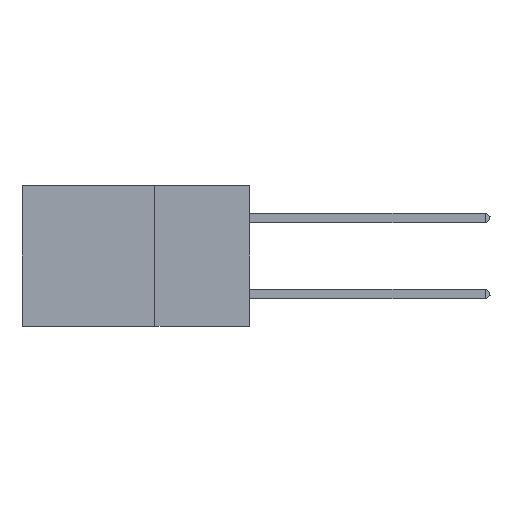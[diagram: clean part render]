
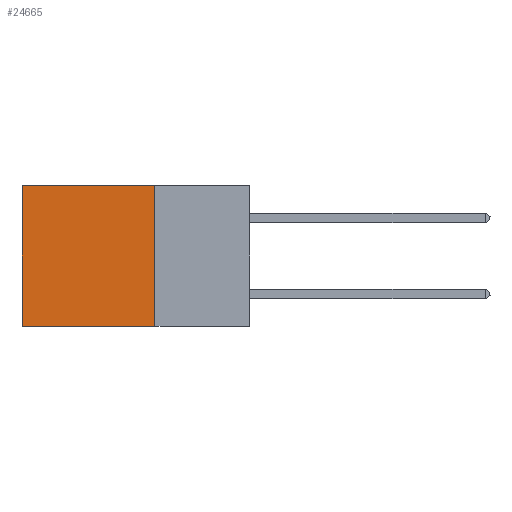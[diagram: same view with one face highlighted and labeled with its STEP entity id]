
A CAD part, left-side view. The second image highlights one B-rep face of the part: STEP entity #24665.
In plain terms, the highlighted planar face has unit normal (-1, 0, 0).
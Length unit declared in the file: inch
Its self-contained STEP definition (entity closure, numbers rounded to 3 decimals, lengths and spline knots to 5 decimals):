
#897 = VECTOR ( 'NONE', #2010, 39.37008 ) ;
#1479 = LINE ( 'NONE', #2839, #30558 ) ;
#2004 = EDGE_CURVE ( 'NONE', #9239, #19953, #13859, .T. ) ;
#2010 = DIRECTION ( 'NONE',  ( 0., 1., 0. ) ) ;
#2092 = ORIENTED_EDGE ( 'NONE', *, *, #23408, .T. ) ;
#2839 = CARTESIAN_POINT ( 'NONE',  ( 0.2875, 0.25, 0. ) ) ;
#2875 = DIRECTION ( 'NONE',  ( 0., 0., -1. ) ) ;
#5859 = DIRECTION ( 'NONE',  ( 0., 0., -1. ) ) ;
#5876 = DIRECTION ( 'NONE',  ( 0., 1., 0. ) ) ;
#7323 = FACE_OUTER_BOUND ( 'NONE', #34072, .T. ) ;
#7855 = VERTEX_POINT ( 'NONE', #29231 ) ;
#8497 = CARTESIAN_POINT ( 'NONE',  ( 0.2875, 0.6, 0. ) ) ;
#8608 = DIRECTION ( 'NONE',  ( 1., 0., 0. ) ) ;
#9239 = VERTEX_POINT ( 'NONE', #19517 ) ;
#10896 = AXIS2_PLACEMENT_3D ( 'NONE', #11439, #8608, #11318 ) ;
#11318 = DIRECTION ( 'NONE',  ( 0., 0., -1. ) ) ;
#11420 = LINE ( 'NONE', #18913, #19392 ) ;
#11439 = CARTESIAN_POINT ( 'NONE',  ( 0.2875, 0.25, 0. ) ) ;
#11648 = CARTESIAN_POINT ( 'NONE',  ( 0.2875, 0.6, -0.37 ) ) ;
#13146 = ORIENTED_EDGE ( 'NONE', *, *, #20541, .F. ) ;
#13859 = LINE ( 'NONE', #31436, #897 ) ;
#18913 = CARTESIAN_POINT ( 'NONE',  ( 0.2875, 0.25, 0. ) ) ;
#19392 = VECTOR ( 'NONE', #5859, 39.37008 ) ;
#19517 = CARTESIAN_POINT ( 'NONE',  ( 0.2875, 0.25, -0.37 ) ) ;
#19953 = VERTEX_POINT ( 'NONE', #11648 ) ;
#20541 = EDGE_CURVE ( 'NONE', #22060, #9239, #11420, .T. ) ;
#21771 = ORIENTED_EDGE ( 'NONE', *, *, #28564, .T. ) ;
#22060 = VERTEX_POINT ( 'NONE', #31339 ) ;
#23408 = EDGE_CURVE ( 'NONE', #7855, #19953, #28926, .T. ) ;
#24665 = ADVANCED_FACE ( 'NONE', ( #7323 ), #30069, .F. ) ;
#27667 = VECTOR ( 'NONE', #2875, 39.37008 ) ;
#28564 = EDGE_CURVE ( 'NONE', #22060, #7855, #1479, .T. ) ;
#28854 = ORIENTED_EDGE ( 'NONE', *, *, #2004, .F. ) ;
#28926 = LINE ( 'NONE', #8497, #27667 ) ;
#29231 = CARTESIAN_POINT ( 'NONE',  ( 0.2875, 0.6, 0. ) ) ;
#30069 = PLANE ( 'NONE',  #10896 ) ;
#30558 = VECTOR ( 'NONE', #5876, 39.37008 ) ;
#31339 = CARTESIAN_POINT ( 'NONE',  ( 0.2875, 0.25, 0. ) ) ;
#31436 = CARTESIAN_POINT ( 'NONE',  ( 0.2875, 0.25, -0.37 ) ) ;
#34072 = EDGE_LOOP ( 'NONE', ( #2092, #28854, #13146, #21771 ) ) ;
